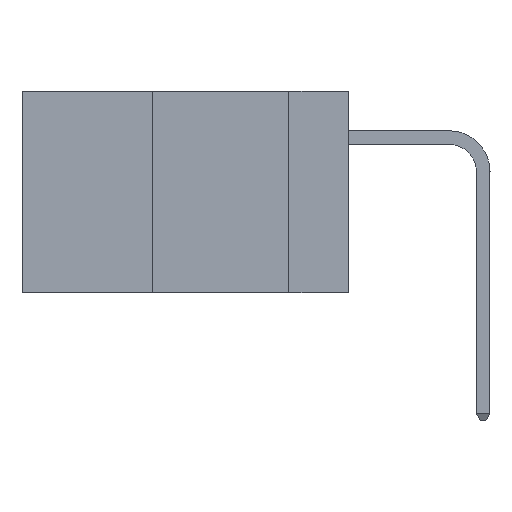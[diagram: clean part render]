
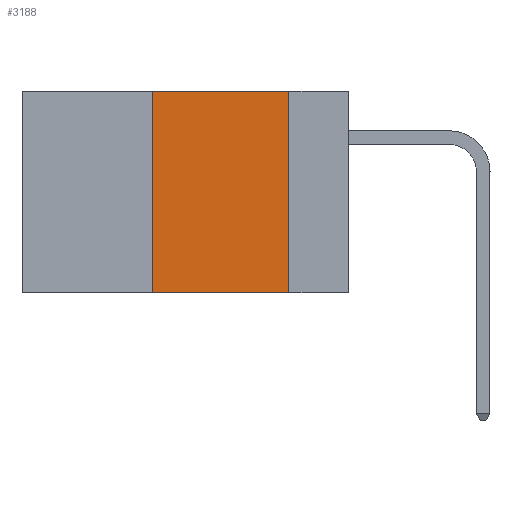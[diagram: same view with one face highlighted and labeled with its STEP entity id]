
A CAD part, left-side view. The second image highlights one B-rep face of the part: STEP entity #3188.
In plain terms, the highlighted planar face has unit normal (-1, 0, 0).
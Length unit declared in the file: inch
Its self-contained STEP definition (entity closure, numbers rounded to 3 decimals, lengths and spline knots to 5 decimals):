
#336 = CARTESIAN_POINT ( 'NONE',  ( 0., 0.11, -0.37 ) ) ;
#991 = CARTESIAN_POINT ( 'NONE',  ( 0., 0.11, 0. ) ) ;
#1291 = VECTOR ( 'NONE', #18819, 39.37008 ) ;
#2030 = ORIENTED_EDGE ( 'NONE', *, *, #6942, .F. ) ;
#2043 = CARTESIAN_POINT ( 'NONE',  ( 0., 0.6, 0. ) ) ;
#2251 = ORIENTED_EDGE ( 'NONE', *, *, #9248, .F. ) ;
#2748 = CARTESIAN_POINT ( 'NONE',  ( 0., 0.36, 0. ) ) ;
#2888 = DIRECTION ( 'NONE',  ( 0., 0., -1. ) ) ;
#3003 = ORIENTED_EDGE ( 'NONE', *, *, #14187, .F. ) ;
#3188 = ADVANCED_FACE ( 'NONE', ( #12816 ), #15056, .F. ) ;
#3407 = VECTOR ( 'NONE', #3471, 39.37008 ) ;
#3471 = DIRECTION ( 'NONE',  ( 0., -1., 0. ) ) ;
#3939 = DIRECTION ( 'NONE',  ( 1., 0., 0. ) ) ;
#4100 = CARTESIAN_POINT ( 'NONE',  ( 0., 0.6, 0. ) ) ;
#4127 = LINE ( 'NONE', #2748, #22945 ) ;
#4128 = CARTESIAN_POINT ( 'NONE',  ( 0., 0.36, -0.37 ) ) ;
#6942 = EDGE_CURVE ( 'NONE', #11135, #22894, #13920, .T. ) ;
#8511 = EDGE_CURVE ( 'NONE', #8629, #22894, #17598, .T. ) ;
#8629 = VERTEX_POINT ( 'NONE', #4128 ) ;
#8661 = EDGE_LOOP ( 'NONE', ( #2030, #2251, #3003, #19530 ) ) ;
#9248 = EDGE_CURVE ( 'NONE', #21754, #11135, #11247, .T. ) ;
#11135 = VERTEX_POINT ( 'NONE', #18721 ) ;
#11247 = LINE ( 'NONE', #4100, #1291 ) ;
#12816 = FACE_OUTER_BOUND ( 'NONE', #8661, .T. ) ;
#13920 = LINE ( 'NONE', #991, #18170 ) ;
#14187 = EDGE_CURVE ( 'NONE', #8629, #21754, #4127, .T. ) ;
#14590 = CARTESIAN_POINT ( 'NONE',  ( 0., 0.6, -0.37 ) ) ;
#14690 = CARTESIAN_POINT ( 'NONE',  ( 0., 0.36, 0. ) ) ;
#15056 = PLANE ( 'NONE',  #17621 ) ;
#16905 = DIRECTION ( 'NONE',  ( 0., 0., -1. ) ) ;
#17574 = DIRECTION ( 'NONE',  ( 0., 0., 1. ) ) ;
#17598 = LINE ( 'NONE', #14590, #3407 ) ;
#17621 = AXIS2_PLACEMENT_3D ( 'NONE', #2043, #3939, #16905 ) ;
#18170 = VECTOR ( 'NONE', #2888, 39.37008 ) ;
#18721 = CARTESIAN_POINT ( 'NONE',  ( 0., 0.11, 0. ) ) ;
#18819 = DIRECTION ( 'NONE',  ( 0., -1., 0. ) ) ;
#19530 = ORIENTED_EDGE ( 'NONE', *, *, #8511, .T. ) ;
#21754 = VERTEX_POINT ( 'NONE', #14690 ) ;
#22894 = VERTEX_POINT ( 'NONE', #336 ) ;
#22945 = VECTOR ( 'NONE', #17574, 39.37008 ) ;
